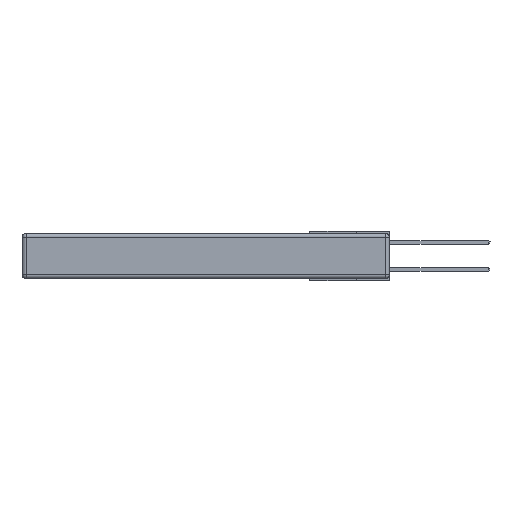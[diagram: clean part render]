
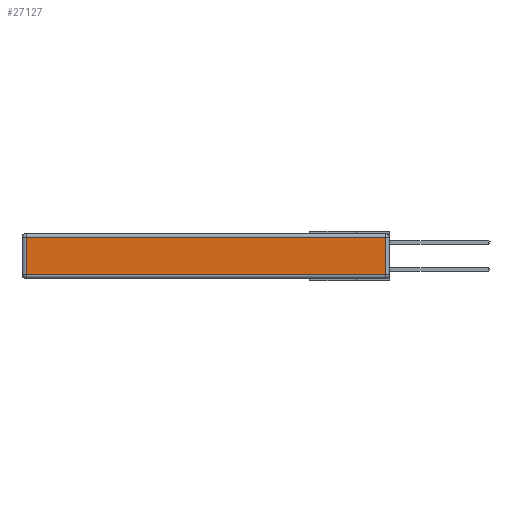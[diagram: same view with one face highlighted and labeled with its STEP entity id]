
A CAD part, left-side view. The second image highlights one B-rep face of the part: STEP entity #27127.
In plain terms, the highlighted planar face has unit normal (-1, 0, 0).
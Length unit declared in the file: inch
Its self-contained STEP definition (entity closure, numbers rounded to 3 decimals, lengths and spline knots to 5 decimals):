
#724 = DIRECTION ( 'NONE',  ( 0., 0., 1. ) ) ;
#2752 = EDGE_CURVE ( 'NONE', #13097, #18005, #25646, .T. ) ;
#2966 = CARTESIAN_POINT ( 'NONE',  ( 0., 0., -0.343 ) ) ;
#3084 = CARTESIAN_POINT ( 'NONE',  ( 0., 0.03, -0.343 ) ) ;
#3110 = DIRECTION ( 'NONE',  ( 0., 0., -1. ) ) ;
#3467 = ORIENTED_EDGE ( 'NONE', *, *, #22988, .T. ) ;
#3486 = CARTESIAN_POINT ( 'NONE',  ( 0., 0.03, -0.03 ) ) ;
#3735 = EDGE_LOOP ( 'NONE', ( #21047, #15351, #6830, #3467 ) ) ;
#5284 = VERTEX_POINT ( 'NONE', #15159 ) ;
#6830 = ORIENTED_EDGE ( 'NONE', *, *, #12100, .T. ) ;
#7516 = DIRECTION ( 'NONE',  ( 0., 0., 1. ) ) ;
#7590 = DIRECTION ( 'NONE',  ( -1., 0., 0. ) ) ;
#9734 = LINE ( 'NONE', #23061, #27467 ) ;
#12100 = EDGE_CURVE ( 'NONE', #20106, #5284, #21050, .T. ) ;
#12453 = EDGE_CURVE ( 'NONE', #18005, #20106, #18741, .T. ) ;
#13097 = VERTEX_POINT ( 'NONE', #28462 ) ;
#13767 = VECTOR ( 'NONE', #25658, 39.37008 ) ;
#15159 = CARTESIAN_POINT ( 'NONE',  ( 0., 2.72, -0.03 ) ) ;
#15351 = ORIENTED_EDGE ( 'NONE', *, *, #12453, .T. ) ;
#18005 = VERTEX_POINT ( 'NONE', #20205 ) ;
#18691 = PLANE ( 'NONE',  #28721 ) ;
#18741 = LINE ( 'NONE', #3084, #20654 ) ;
#19851 = DIRECTION ( 'NONE',  ( 0., 1., 0. ) ) ;
#20106 = VERTEX_POINT ( 'NONE', #3486 ) ;
#20205 = CARTESIAN_POINT ( 'NONE',  ( 0., 0.03, -0.313 ) ) ;
#20654 = VECTOR ( 'NONE', #7516, 39.37008 ) ;
#20789 = CARTESIAN_POINT ( 'NONE',  ( 0., 0., -0.313 ) ) ;
#21047 = ORIENTED_EDGE ( 'NONE', *, *, #2752, .T. ) ;
#21050 = LINE ( 'NONE', #24270, #23115 ) ;
#22988 = EDGE_CURVE ( 'NONE', #5284, #13097, #9734, .T. ) ;
#23061 = CARTESIAN_POINT ( 'NONE',  ( 0., 2.72, -0.343 ) ) ;
#23115 = VECTOR ( 'NONE', #19851, 39.37008 ) ;
#24270 = CARTESIAN_POINT ( 'NONE',  ( 0., 2.75, -0.03 ) ) ;
#25646 = LINE ( 'NONE', #20789, #13767 ) ;
#25658 = DIRECTION ( 'NONE',  ( 0., -1., 0. ) ) ;
#27127 = ADVANCED_FACE ( 'NONE', ( #28840 ), #18691, .T. ) ;
#27467 = VECTOR ( 'NONE', #3110, 39.37008 ) ;
#28462 = CARTESIAN_POINT ( 'NONE',  ( 0., 2.72, -0.313 ) ) ;
#28721 = AXIS2_PLACEMENT_3D ( 'NONE', #2966, #7590, #724 ) ;
#28840 = FACE_OUTER_BOUND ( 'NONE', #3735, .T. ) ;
